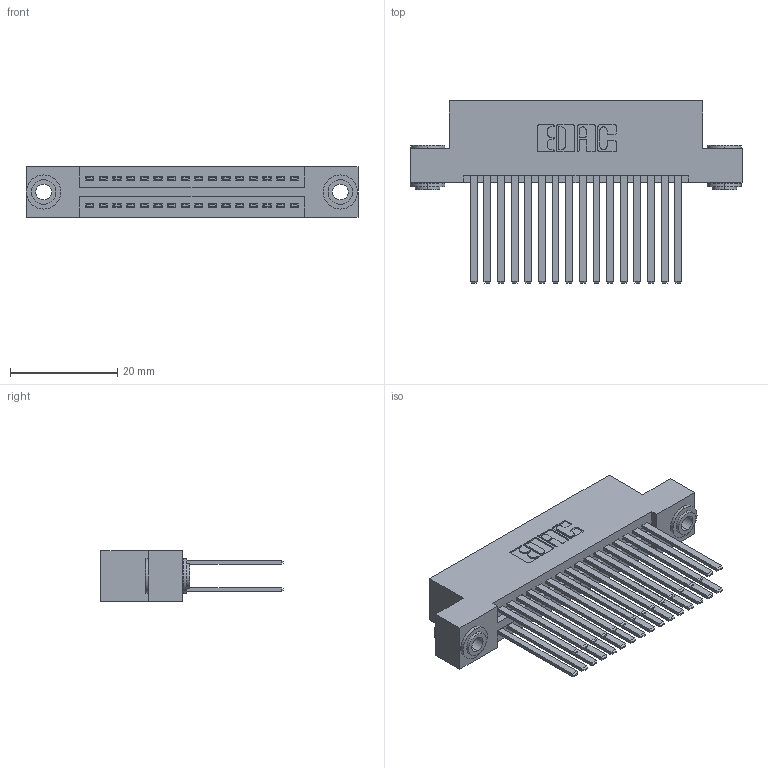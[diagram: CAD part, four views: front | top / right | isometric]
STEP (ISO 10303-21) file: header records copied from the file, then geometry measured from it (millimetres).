
FILE_DESCRIPTION (( 'STEP AP203' ), '1' );
FILE_NAME ('345-032-544-203.STEP', '2018-08-24T07:54:06', ( '' ), ( '' ), 'SwSTEP 2.0', 'SolidWorks 2016', '' );
FILE_SCHEMA (( 'CONFIG_CONTROL_DESIGN' ));
Length unit declared in the file: inch
Products named in the file (4): 345 Part_Flush Mounting Lugs - 0.156 Dia-TH; 345-292-001_345-293-144; 345-250-002_345-250-002-102; 345-032-544-203
Assembly tree (35 placements, depth 2):
  345-032-544-203
    345 Part_Flush Mounting Lugs - 0.156 Dia-TH
    345-292-001_345-293-144  x32
    345-250-002_345-250-002-102  x2
Bounding box: 61.85 x 33.96 x 9.4 mm (x, y, z)
Volume: 6234.7 mm3; surface area: 10232 mm2
Topology: 35 solids, 35 shells, 1572 faces, 4609 edges, 3026 vertices
Faces by surface type: plane 1018, cylinder 546, cone 8
Entity records: 16520 total; most frequent: CARTESIAN_POINT 2767, ORIENTED_EDGE 2694, DIRECTION 2501, EDGE_CURVE 1347, VECTOR 1131, LINE 1131, VERTEX_POINT 894, AXIS2_PLACEMENT_3D 685
